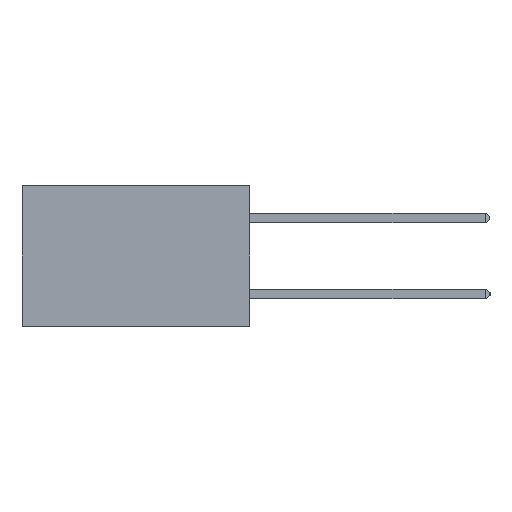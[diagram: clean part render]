
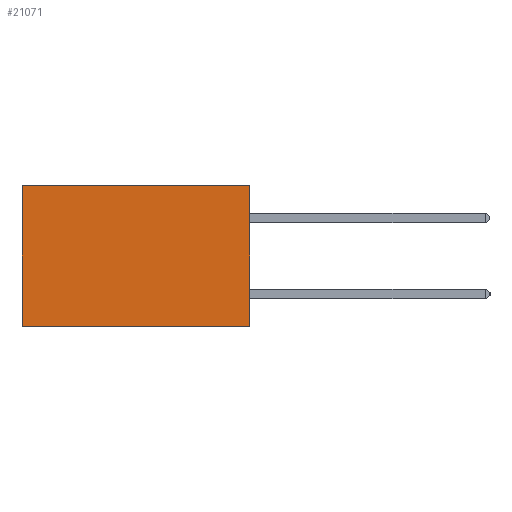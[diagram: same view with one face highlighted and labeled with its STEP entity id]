
A CAD part, left-side view. The second image highlights one B-rep face of the part: STEP entity #21071.
In plain terms, the highlighted planar face has unit normal (-1, 0, 0).
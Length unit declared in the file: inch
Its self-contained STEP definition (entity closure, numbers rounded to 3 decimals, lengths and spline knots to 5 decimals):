
#727 = EDGE_CURVE ( 'NONE', #16315, #7843, #16182, .T. ) ;
#809 = VECTOR ( 'NONE', #26869, 39.37008 ) ;
#2282 = LINE ( 'NONE', #12854, #809 ) ;
#2413 = VECTOR ( 'NONE', #9707, 39.37008 ) ;
#4641 = CARTESIAN_POINT ( 'NONE',  ( 0.2875, 0.6, -0.37 ) ) ;
#5899 = LINE ( 'NONE', #25368, #2413 ) ;
#6167 = EDGE_CURVE ( 'NONE', #19597, #14990, #5899, .T. ) ;
#6347 = CARTESIAN_POINT ( 'NONE',  ( 0.2875, 0., 0. ) ) ;
#6537 = ORIENTED_EDGE ( 'NONE', *, *, #727, .F. ) ;
#7277 = CARTESIAN_POINT ( 'NONE',  ( 0.2875, 0., 0. ) ) ;
#7427 = ORIENTED_EDGE ( 'NONE', *, *, #25416, .F. ) ;
#7843 = VERTEX_POINT ( 'NONE', #4641 ) ;
#8495 = CARTESIAN_POINT ( 'NONE',  ( 0.2875, 0., 0. ) ) ;
#9480 = LINE ( 'NONE', #7277, #13904 ) ;
#9707 = DIRECTION ( 'NONE',  ( 0., 1., 0. ) ) ;
#9997 = ORIENTED_EDGE ( 'NONE', *, *, #35770, .T. ) ;
#12854 = CARTESIAN_POINT ( 'NONE',  ( 0.2875, 0.6, 0. ) ) ;
#13467 = CARTESIAN_POINT ( 'NONE',  ( 0.2875, 0., -0.37 ) ) ;
#13904 = VECTOR ( 'NONE', #15633, 39.37008 ) ;
#13920 = CARTESIAN_POINT ( 'NONE',  ( 0.2875, 0., -0.37 ) ) ;
#14990 = VERTEX_POINT ( 'NONE', #24843 ) ;
#15633 = DIRECTION ( 'NONE',  ( 0., 0., -1. ) ) ;
#16182 = LINE ( 'NONE', #13467, #20324 ) ;
#16315 = VERTEX_POINT ( 'NONE', #13920 ) ;
#17434 = DIRECTION ( 'NONE',  ( 0., 0., -1. ) ) ;
#19597 = VERTEX_POINT ( 'NONE', #8495 ) ;
#20324 = VECTOR ( 'NONE', #24377, 39.37008 ) ;
#20988 = AXIS2_PLACEMENT_3D ( 'NONE', #6347, #34327, #17434 ) ;
#21071 = ADVANCED_FACE ( 'NONE', ( #23263 ), #31087, .F. ) ;
#23263 = FACE_OUTER_BOUND ( 'NONE', #34242, .T. ) ;
#24377 = DIRECTION ( 'NONE',  ( 0., 1., 0. ) ) ;
#24843 = CARTESIAN_POINT ( 'NONE',  ( 0.2875, 0.6, 0. ) ) ;
#25368 = CARTESIAN_POINT ( 'NONE',  ( 0.2875, 0., 0. ) ) ;
#25416 = EDGE_CURVE ( 'NONE', #19597, #16315, #9480, .T. ) ;
#25437 = ORIENTED_EDGE ( 'NONE', *, *, #6167, .T. ) ;
#26869 = DIRECTION ( 'NONE',  ( 0., 0., -1. ) ) ;
#31087 = PLANE ( 'NONE',  #20988 ) ;
#34242 = EDGE_LOOP ( 'NONE', ( #9997, #6537, #7427, #25437 ) ) ;
#34327 = DIRECTION ( 'NONE',  ( 1., 0., 0. ) ) ;
#35770 = EDGE_CURVE ( 'NONE', #14990, #7843, #2282, .T. ) ;
